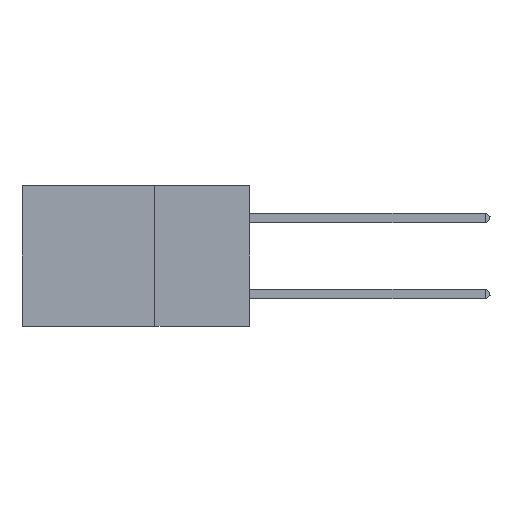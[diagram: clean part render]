
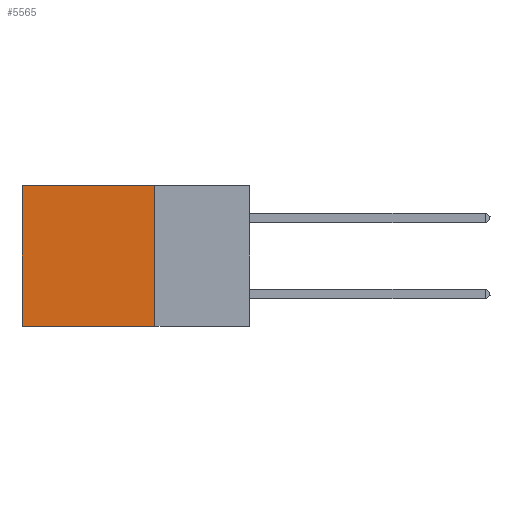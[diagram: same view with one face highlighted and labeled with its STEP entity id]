
A CAD part, left-side view. The second image highlights one B-rep face of the part: STEP entity #5565.
In plain terms, the highlighted planar face has unit normal (-1, 0, 0).
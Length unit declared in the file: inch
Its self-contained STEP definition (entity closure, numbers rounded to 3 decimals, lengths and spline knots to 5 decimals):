
#347 = VERTEX_POINT ( 'NONE', #30004 ) ;
#4123 = ORIENTED_EDGE ( 'NONE', *, *, #20548, .T. ) ;
#5183 = VECTOR ( 'NONE', #14208, 39.37008 ) ;
#5565 = ADVANCED_FACE ( 'NONE', ( #6136 ), #8731, .F. ) ;
#5787 = AXIS2_PLACEMENT_3D ( 'NONE', #11407, #21219, #6626 ) ;
#6136 = FACE_OUTER_BOUND ( 'NONE', #14367, .T. ) ;
#6626 = DIRECTION ( 'NONE',  ( 0., 0., -1. ) ) ;
#6787 = VECTOR ( 'NONE', #10135, 39.37008 ) ;
#8297 = LINE ( 'NONE', #12307, #6787 ) ;
#8731 = PLANE ( 'NONE',  #5787 ) ;
#10135 = DIRECTION ( 'NONE',  ( 0., 0., -1. ) ) ;
#10312 = CARTESIAN_POINT ( 'NONE',  ( 0.2875, 0.25, 0. ) ) ;
#11064 = CARTESIAN_POINT ( 'NONE',  ( 0.2875, 0.25, -0.37 ) ) ;
#11284 = VECTOR ( 'NONE', #16730, 39.37008 ) ;
#11291 = EDGE_CURVE ( 'NONE', #347, #30090, #20085, .T. ) ;
#11407 = CARTESIAN_POINT ( 'NONE',  ( 0.2875, 0.25, 0. ) ) ;
#12307 = CARTESIAN_POINT ( 'NONE',  ( 0.2875, 0.25, 0. ) ) ;
#13055 = LINE ( 'NONE', #10312, #28669 ) ;
#13221 = LINE ( 'NONE', #13887, #5183 ) ;
#13887 = CARTESIAN_POINT ( 'NONE',  ( 0.2875, 0.25, -0.37 ) ) ;
#14208 = DIRECTION ( 'NONE',  ( 0., 1., 0. ) ) ;
#14367 = EDGE_LOOP ( 'NONE', ( #28199, #24210, #17869, #4123 ) ) ;
#14440 = VERTEX_POINT ( 'NONE', #11064 ) ;
#16730 = DIRECTION ( 'NONE',  ( 0., 0., -1. ) ) ;
#16887 = EDGE_CURVE ( 'NONE', #14440, #30090, #13221, .T. ) ;
#17260 = DIRECTION ( 'NONE',  ( 0., 1., 0. ) ) ;
#17869 = ORIENTED_EDGE ( 'NONE', *, *, #22906, .F. ) ;
#20085 = LINE ( 'NONE', #21399, #11284 ) ;
#20548 = EDGE_CURVE ( 'NONE', #23067, #347, #13055, .T. ) ;
#21219 = DIRECTION ( 'NONE',  ( 1., 0., 0. ) ) ;
#21399 = CARTESIAN_POINT ( 'NONE',  ( 0.2875, 0.6, 0. ) ) ;
#22906 = EDGE_CURVE ( 'NONE', #23067, #14440, #8297, .T. ) ;
#23067 = VERTEX_POINT ( 'NONE', #25467 ) ;
#24210 = ORIENTED_EDGE ( 'NONE', *, *, #16887, .F. ) ;
#25467 = CARTESIAN_POINT ( 'NONE',  ( 0.2875, 0.25, 0. ) ) ;
#26112 = CARTESIAN_POINT ( 'NONE',  ( 0.2875, 0.6, -0.37 ) ) ;
#28199 = ORIENTED_EDGE ( 'NONE', *, *, #11291, .T. ) ;
#28669 = VECTOR ( 'NONE', #17260, 39.37008 ) ;
#30004 = CARTESIAN_POINT ( 'NONE',  ( 0.2875, 0.6, 0. ) ) ;
#30090 = VERTEX_POINT ( 'NONE', #26112 ) ;
